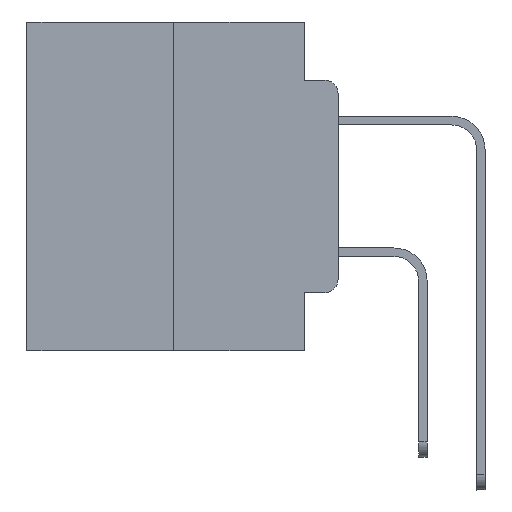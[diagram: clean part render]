
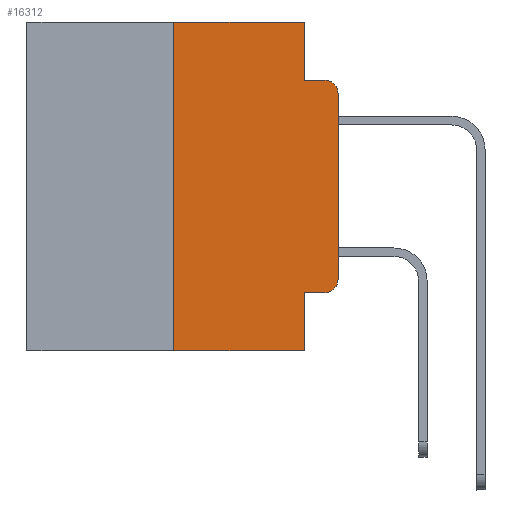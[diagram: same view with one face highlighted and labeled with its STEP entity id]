
A CAD part, left-side view. The second image highlights one B-rep face of the part: STEP entity #16312.
In plain terms, the highlighted planar face has unit normal (-1, 0, 0).
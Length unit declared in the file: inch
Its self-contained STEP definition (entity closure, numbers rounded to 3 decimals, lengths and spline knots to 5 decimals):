
#468 = DIRECTION ( 'NONE',  ( -1., 0., 0. ) ) ;
#831 = AXIS2_PLACEMENT_3D ( 'NONE', #25208, #5311, #20946 ) ;
#1389 = ORIENTED_EDGE ( 'NONE', *, *, #26960, .T. ) ;
#1533 = AXIS2_PLACEMENT_3D ( 'NONE', #14074, #468, #16308 ) ;
#1627 = CARTESIAN_POINT ( 'NONE',  ( 0., 0.051, 0. ) ) ;
#1763 = DIRECTION ( 'NONE',  ( 0., 0., -1. ) ) ;
#1924 = LINE ( 'NONE', #1627, #19222 ) ;
#2185 = VERTEX_POINT ( 'NONE', #17240 ) ;
#2815 = VERTEX_POINT ( 'NONE', #17200 ) ;
#3937 = DIRECTION ( 'NONE',  ( 0., 0., -1. ) ) ;
#4386 = VERTEX_POINT ( 'NONE', #11556 ) ;
#5311 = DIRECTION ( 'NONE',  ( 1., 0., 0. ) ) ;
#6343 = VECTOR ( 'NONE', #25141, 39.37008 ) ;
#6994 = VECTOR ( 'NONE', #23390, 39.37008 ) ;
#7154 = ORIENTED_EDGE ( 'NONE', *, *, #25734, .T. ) ;
#7352 = VERTEX_POINT ( 'NONE', #26859 ) ;
#8426 = LINE ( 'NONE', #21211, #6994 ) ;
#9414 = CARTESIAN_POINT ( 'NONE',  ( 0., 0., 0. ) ) ;
#9524 = LINE ( 'NONE', #25434, #19955 ) ;
#10727 = LINE ( 'NONE', #9414, #27572 ) ;
#11556 = CARTESIAN_POINT ( 'NONE',  ( 0., 0.051, -0.5 ) ) ;
#12046 = ORIENTED_EDGE ( 'NONE', *, *, #26166, .F. ) ;
#13699 = CARTESIAN_POINT ( 'NONE',  ( 0., 0.051, -0.0885 ) ) ;
#13888 = DIRECTION ( 'NONE',  ( 0., 0., 1. ) ) ;
#13914 = AXIS2_PLACEMENT_3D ( 'NONE', #28434, #15354, #1763 ) ;
#14074 = CARTESIAN_POINT ( 'NONE',  ( 0., 0.02, -0.3915 ) ) ;
#14197 = CARTESIAN_POINT ( 'NONE',  ( 0., 0.051, -0.0885 ) ) ;
#14459 = DIRECTION ( 'NONE',  ( 0., 0., 1. ) ) ;
#14514 = DIRECTION ( 'NONE',  ( 0., -1., 0. ) ) ;
#14823 = ORIENTED_EDGE ( 'NONE', *, *, #17154, .T. ) ;
#15354 = DIRECTION ( 'NONE',  ( -1., 0., 0. ) ) ;
#16109 = VERTEX_POINT ( 'NONE', #18091 ) ;
#16203 = ORIENTED_EDGE ( 'NONE', *, *, #24132, .T. ) ;
#16308 = DIRECTION ( 'NONE',  ( 0., 0., -1. ) ) ;
#16312 = ADVANCED_FACE ( 'NONE', ( #19120 ), #27390, .F. ) ;
#17154 = EDGE_CURVE ( 'NONE', #23489, #26037, #10727, .T. ) ;
#17200 = CARTESIAN_POINT ( 'NONE',  ( 0., 0.25, 0. ) ) ;
#17240 = CARTESIAN_POINT ( 'NONE',  ( 0., 0.051, -0.4115 ) ) ;
#17593 = VECTOR ( 'NONE', #25338, 39.37008 ) ;
#17739 = LINE ( 'NONE', #21130, #23553 ) ;
#18091 = CARTESIAN_POINT ( 'NONE',  ( 0., 0.25, -0.5 ) ) ;
#18176 = CARTESIAN_POINT ( 'NONE',  ( 0., 0.051, 0. ) ) ;
#18403 = VERTEX_POINT ( 'NONE', #27526 ) ;
#18418 = EDGE_CURVE ( 'NONE', #2815, #28293, #9524, .T. ) ;
#19120 = FACE_OUTER_BOUND ( 'NONE', #23378, .T. ) ;
#19222 = VECTOR ( 'NONE', #3937, 39.37008 ) ;
#19452 = CARTESIAN_POINT ( 'NONE',  ( 0., 0., -0.3915 ) ) ;
#19759 = VERTEX_POINT ( 'NONE', #13699 ) ;
#19955 = VECTOR ( 'NONE', #14514, 39.37008 ) ;
#20363 = DIRECTION ( 'NONE',  ( 0., 0., -1. ) ) ;
#20946 = DIRECTION ( 'NONE',  ( 0., 0., -1. ) ) ;
#21075 = ORIENTED_EDGE ( 'NONE', *, *, #21902, .F. ) ;
#21130 = CARTESIAN_POINT ( 'NONE',  ( 0., 0.25, 0. ) ) ;
#21211 = CARTESIAN_POINT ( 'NONE',  ( 0., 0.473, -0.5 ) ) ;
#21342 = CARTESIAN_POINT ( 'NONE',  ( 0., 0.051, 0. ) ) ;
#21715 = EDGE_CURVE ( 'NONE', #2185, #4386, #22534, .T. ) ;
#21902 = EDGE_CURVE ( 'NONE', #16109, #2815, #17739, .T. ) ;
#22116 = ORIENTED_EDGE ( 'NONE', *, *, #21715, .F. ) ;
#22118 = CARTESIAN_POINT ( 'NONE',  ( 0., 0., -0.1085 ) ) ;
#22492 = EDGE_CURVE ( 'NONE', #7352, #23489, #23168, .T. ) ;
#22534 = LINE ( 'NONE', #18176, #27617 ) ;
#23168 = CIRCLE ( 'NONE', #1533, 0.02 ) ;
#23177 = CARTESIAN_POINT ( 'NONE',  ( 0., 0.051, -0.4115 ) ) ;
#23378 = EDGE_LOOP ( 'NONE', ( #14823, #16203, #12046, #25810, #24125, #21075, #1389, #22116, #7154, #27679 ) ) ;
#23390 = DIRECTION ( 'NONE',  ( 0., -1., 0. ) ) ;
#23408 = LINE ( 'NONE', #23177, #17593 ) ;
#23489 = VERTEX_POINT ( 'NONE', #19452 ) ;
#23553 = VECTOR ( 'NONE', #14459, 39.37008 ) ;
#24125 = ORIENTED_EDGE ( 'NONE', *, *, #18418, .F. ) ;
#24132 = EDGE_CURVE ( 'NONE', #26037, #18403, #26562, .T. ) ;
#24736 = LINE ( 'NONE', #14197, #6343 ) ;
#25141 = DIRECTION ( 'NONE',  ( 0., -1., 0. ) ) ;
#25208 = CARTESIAN_POINT ( 'NONE',  ( 0., 0.473, 0. ) ) ;
#25338 = DIRECTION ( 'NONE',  ( 0., -1., 0. ) ) ;
#25434 = CARTESIAN_POINT ( 'NONE',  ( 0., 0.473, 0. ) ) ;
#25734 = EDGE_CURVE ( 'NONE', #2185, #7352, #23408, .T. ) ;
#25810 = ORIENTED_EDGE ( 'NONE', *, *, #27136, .F. ) ;
#26037 = VERTEX_POINT ( 'NONE', #22118 ) ;
#26166 = EDGE_CURVE ( 'NONE', #19759, #18403, #24736, .T. ) ;
#26562 = CIRCLE ( 'NONE', #13914, 0.02 ) ;
#26859 = CARTESIAN_POINT ( 'NONE',  ( 0., 0.02, -0.4115 ) ) ;
#26960 = EDGE_CURVE ( 'NONE', #16109, #4386, #8426, .T. ) ;
#27136 = EDGE_CURVE ( 'NONE', #28293, #19759, #1924, .T. ) ;
#27390 = PLANE ( 'NONE',  #831 ) ;
#27526 = CARTESIAN_POINT ( 'NONE',  ( 0., 0.02, -0.0885 ) ) ;
#27572 = VECTOR ( 'NONE', #13888, 39.37008 ) ;
#27617 = VECTOR ( 'NONE', #20363, 39.37008 ) ;
#27679 = ORIENTED_EDGE ( 'NONE', *, *, #22492, .T. ) ;
#28293 = VERTEX_POINT ( 'NONE', #21342 ) ;
#28434 = CARTESIAN_POINT ( 'NONE',  ( 0., 0.02, -0.1085 ) ) ;
